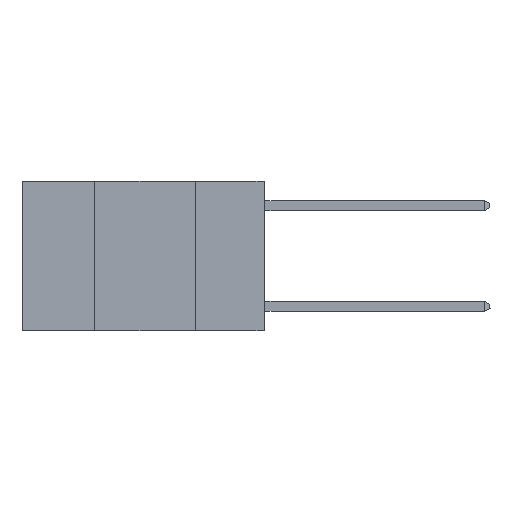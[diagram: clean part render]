
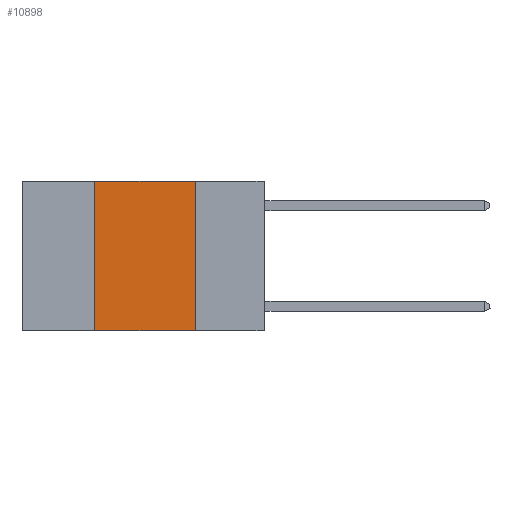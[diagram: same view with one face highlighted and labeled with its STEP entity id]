
A CAD part, left-side view. The second image highlights one B-rep face of the part: STEP entity #10898.
In plain terms, the highlighted planar face has unit normal (-1, 0, 0).
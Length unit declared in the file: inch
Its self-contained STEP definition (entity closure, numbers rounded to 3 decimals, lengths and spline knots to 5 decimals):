
#151 = ORIENTED_EDGE ( 'NONE', *, *, #8100, .T. ) ;
#661 = LINE ( 'NONE', #4136, #12861 ) ;
#878 = VERTEX_POINT ( 'NONE', #13831 ) ;
#1004 = ORIENTED_EDGE ( 'NONE', *, *, #10919, .F. ) ;
#1307 = LINE ( 'NONE', #10289, #4821 ) ;
#1543 = DIRECTION ( 'NONE',  ( 0., -1., 0. ) ) ;
#2708 = EDGE_CURVE ( 'NONE', #878, #6279, #1307, .T. ) ;
#3128 = LINE ( 'NONE', #14408, #7909 ) ;
#3501 = VERTEX_POINT ( 'NONE', #12435 ) ;
#3680 = CARTESIAN_POINT ( 'NONE',  ( 0., 0.6, 0. ) ) ;
#3899 = EDGE_LOOP ( 'NONE', ( #11086, #1004, #10512, #151 ) ) ;
#4136 = CARTESIAN_POINT ( 'NONE',  ( 0., 0.17, 0. ) ) ;
#4821 = VECTOR ( 'NONE', #5695, 39.37008 ) ;
#4844 = PLANE ( 'NONE',  #14001 ) ;
#5695 = DIRECTION ( 'NONE',  ( 0., 0., 1. ) ) ;
#6230 = LINE ( 'NONE', #3680, #6764 ) ;
#6279 = VERTEX_POINT ( 'NONE', #11833 ) ;
#6764 = VECTOR ( 'NONE', #1543, 39.37008 ) ;
#7635 = EDGE_CURVE ( 'NONE', #12606, #3501, #661, .T. ) ;
#7909 = VECTOR ( 'NONE', #13361, 39.37008 ) ;
#8100 = EDGE_CURVE ( 'NONE', #878, #3501, #3128, .T. ) ;
#8203 = FACE_OUTER_BOUND ( 'NONE', #3899, .T. ) ;
#10289 = CARTESIAN_POINT ( 'NONE',  ( 0., 0.42, 0. ) ) ;
#10300 = CARTESIAN_POINT ( 'NONE',  ( 0., 0.17, 0. ) ) ;
#10512 = ORIENTED_EDGE ( 'NONE', *, *, #2708, .F. ) ;
#10898 = ADVANCED_FACE ( 'NONE', ( #8203 ), #4844, .F. ) ;
#10901 = DIRECTION ( 'NONE',  ( 0., 0., -1. ) ) ;
#10919 = EDGE_CURVE ( 'NONE', #6279, #12606, #6230, .T. ) ;
#11086 = ORIENTED_EDGE ( 'NONE', *, *, #7635, .F. ) ;
#11479 = DIRECTION ( 'NONE',  ( 0., 0., -1. ) ) ;
#11633 = CARTESIAN_POINT ( 'NONE',  ( 0., 0.6, 0. ) ) ;
#11833 = CARTESIAN_POINT ( 'NONE',  ( 0., 0.42, 0. ) ) ;
#12435 = CARTESIAN_POINT ( 'NONE',  ( 0., 0.17, -0.37 ) ) ;
#12606 = VERTEX_POINT ( 'NONE', #10300 ) ;
#12861 = VECTOR ( 'NONE', #10901, 39.37008 ) ;
#13361 = DIRECTION ( 'NONE',  ( 0., -1., 0. ) ) ;
#13831 = CARTESIAN_POINT ( 'NONE',  ( 0., 0.42, -0.37 ) ) ;
#13985 = DIRECTION ( 'NONE',  ( 1., 0., 0. ) ) ;
#14001 = AXIS2_PLACEMENT_3D ( 'NONE', #11633, #13985, #11479 ) ;
#14408 = CARTESIAN_POINT ( 'NONE',  ( 0., 0.6, -0.37 ) ) ;
